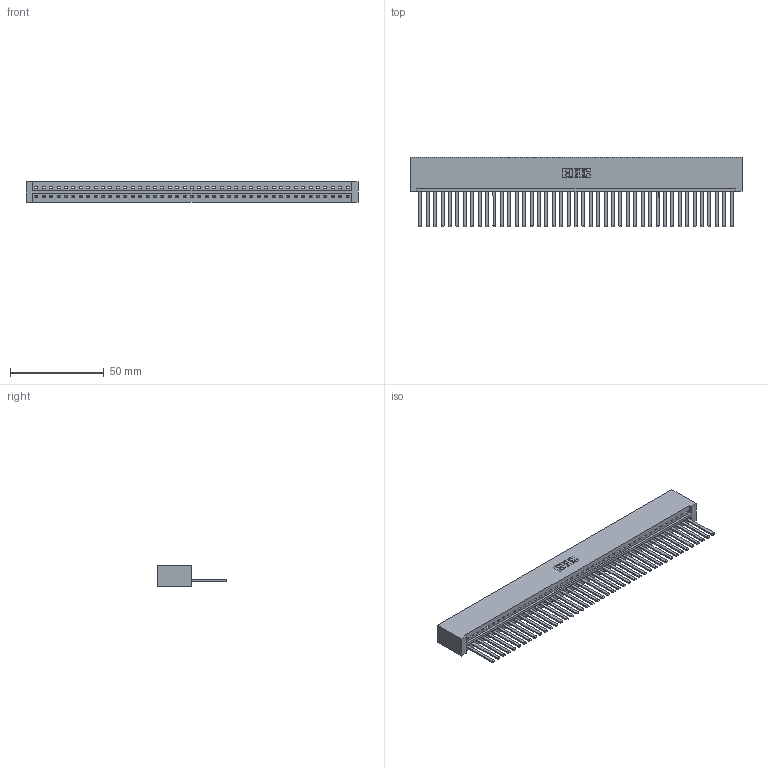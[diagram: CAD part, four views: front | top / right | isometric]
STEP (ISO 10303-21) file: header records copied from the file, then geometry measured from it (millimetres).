
FILE_DESCRIPTION (( 'STEP AP203' ), '1' );
FILE_NAME ('336-043-541-601.STEP', '2020-08-07T23:43:11', ( '' ), ( '' ), 'SwSTEP 2.0', 'SolidWorks 2020', '' );
FILE_SCHEMA (( 'CONFIG_CONTROL_DESIGN' ));
Length unit declared in the file: inch
Products named in the file (3): 336 Part_Lugless; 336-043-541-601; 336-290-001_336-290-541
Assembly tree (44 placements, depth 2):
  336-043-541-601
    336 Part_Lugless
    336-290-001_336-290-541  x43
Bounding box: 177.5 x 37.34 x 11.1 mm (x, y, z)
Volume: 27426.1 mm3; surface area: 29899.4 mm2
Topology: 44 solids, 44 shells, 2256 faces, 6909 edges, 4576 vertices
Faces by surface type: plane 1528, cylinder 728
Entity records: 31276 total; most frequent: CARTESIAN_POINT 5538, ORIENTED_EDGE 5418, DIRECTION 4555, EDGE_CURVE 2709, VECTOR 2585, LINE 2585, VERTEX_POINT 1804, AXIS2_PLACEMENT_3D 985
